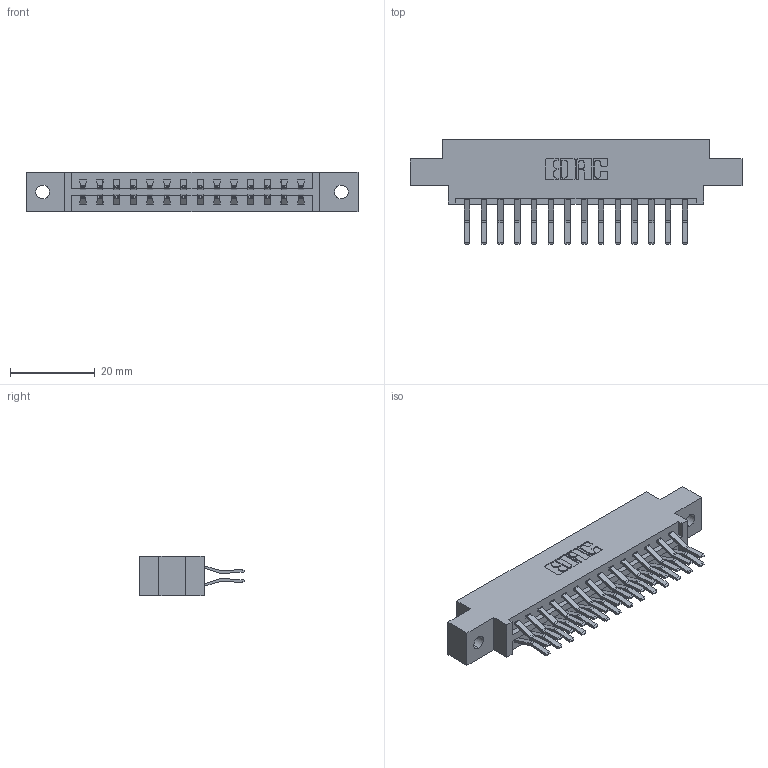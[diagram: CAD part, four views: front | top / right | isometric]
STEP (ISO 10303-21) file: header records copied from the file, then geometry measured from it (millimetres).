
FILE_DESCRIPTION (( 'STEP AP203' ), '1' );
FILE_NAME ('337-028-560-802.STEP', '2018-08-06T12:44:28', ( '' ), ( '' ), 'SwSTEP 2.0', 'SolidWorks 2016', '' );
FILE_SCHEMA (( 'CONFIG_CONTROL_DESIGN' ));
Length unit declared in the file: inch
Products named in the file (3): 337 Part_0.170 Offset - 0.128 Dia; 345-292-001_560 Tail; 337-028-560-802
Assembly tree (29 placements, depth 2):
  337-028-560-802
    337 Part_0.170 Offset - 0.128 Dia
    345-292-001_560 Tail  x28
Bounding box: 78.49 x 24.78 x 9.4 mm (x, y, z)
Volume: 7928.1 mm3; surface area: 9057.1 mm2
Topology: 29 solids, 29 shells, 1686 faces, 4999 edges, 3294 vertices
Faces by surface type: plane 1138, cylinder 548
Entity records: 14699 total; most frequent: CARTESIAN_POINT 2502, ORIENTED_EDGE 2438, DIRECTION 2183, EDGE_CURVE 1219, VECTOR 1087, LINE 1087, VERTEX_POINT 810, AXIS2_PLACEMENT_3D 548
